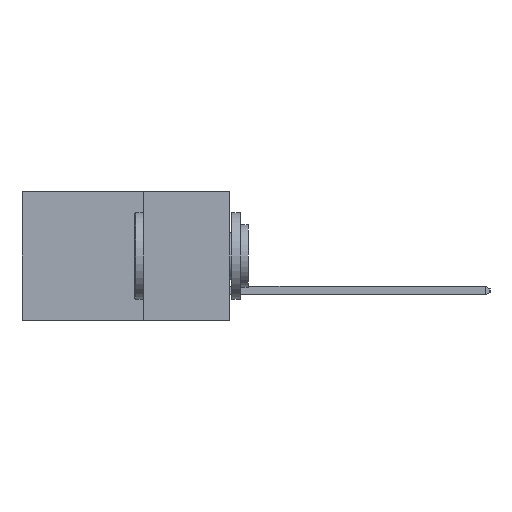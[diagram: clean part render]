
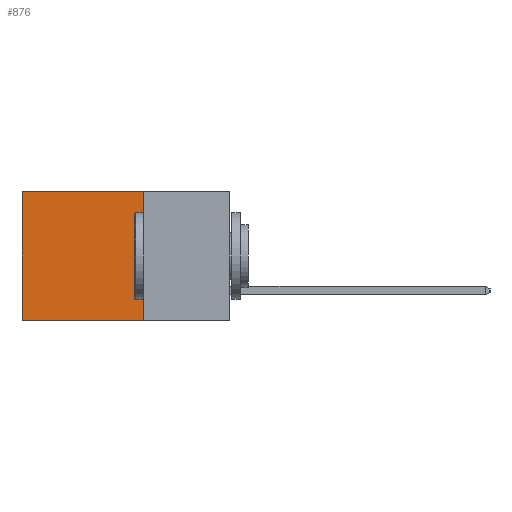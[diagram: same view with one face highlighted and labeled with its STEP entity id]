
A CAD part, left-side view. The second image highlights one B-rep face of the part: STEP entity #876.
In plain terms, the highlighted planar face has unit normal (-1, 0, 0).
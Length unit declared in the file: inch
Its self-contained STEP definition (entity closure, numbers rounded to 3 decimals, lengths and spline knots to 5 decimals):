
#803 = CARTESIAN_POINT ( 'NONE',  ( 0.298, 0.25, 0. ) ) ;
#833 = LINE ( 'NONE', #9248, #12348 ) ;
#876 = ADVANCED_FACE ( 'NONE', ( #4992 ), #11235, .F. ) ;
#1452 = EDGE_CURVE ( 'NONE', #3999, #16987, #19710, .T. ) ;
#1495 = EDGE_LOOP ( 'NONE', ( #12972, #16154, #17252, #1622 ) ) ;
#1622 = ORIENTED_EDGE ( 'NONE', *, *, #1452, .T. ) ;
#2278 = CARTESIAN_POINT ( 'NONE',  ( 0.298, 0.25, 0. ) ) ;
#2587 = VERTEX_POINT ( 'NONE', #16892 ) ;
#3330 = CARTESIAN_POINT ( 'NONE',  ( 0.298, 0.25, -0.37 ) ) ;
#3335 = CARTESIAN_POINT ( 'NONE',  ( 0.298, 0.25, -0.37 ) ) ;
#3428 = VECTOR ( 'NONE', #10988, 39.37008 ) ;
#3999 = VERTEX_POINT ( 'NONE', #2278 ) ;
#4008 = LINE ( 'NONE', #3335, #11269 ) ;
#4130 = DIRECTION ( 'NONE',  ( 0., 0., -1. ) ) ;
#4992 = FACE_OUTER_BOUND ( 'NONE', #1495, .T. ) ;
#5672 = CARTESIAN_POINT ( 'NONE',  ( 0.298, 0.6, 0. ) ) ;
#7982 = DIRECTION ( 'NONE',  ( 1., 0., 0. ) ) ;
#8150 = DIRECTION ( 'NONE',  ( 0., 0., -1. ) ) ;
#8777 = CARTESIAN_POINT ( 'NONE',  ( 0.298, 0.6, 0. ) ) ;
#9248 = CARTESIAN_POINT ( 'NONE',  ( 0.298, 0.25, 0. ) ) ;
#10777 = DIRECTION ( 'NONE',  ( 0., 0., -1. ) ) ;
#10870 = LINE ( 'NONE', #5672, #18910 ) ;
#10988 = DIRECTION ( 'NONE',  ( 0., 1., 0. ) ) ;
#11235 = PLANE ( 'NONE',  #14724 ) ;
#11269 = VECTOR ( 'NONE', #12668, 39.37008 ) ;
#11932 = EDGE_CURVE ( 'NONE', #15998, #2587, #4008, .T. ) ;
#12348 = VECTOR ( 'NONE', #10777, 39.37008 ) ;
#12668 = DIRECTION ( 'NONE',  ( 0., 1., 0. ) ) ;
#12972 = ORIENTED_EDGE ( 'NONE', *, *, #17650, .T. ) ;
#13404 = CARTESIAN_POINT ( 'NONE',  ( 0.298, 0.25, 0. ) ) ;
#14142 = EDGE_CURVE ( 'NONE', #3999, #15998, #833, .T. ) ;
#14724 = AXIS2_PLACEMENT_3D ( 'NONE', #13404, #7982, #8150 ) ;
#15998 = VERTEX_POINT ( 'NONE', #3330 ) ;
#16154 = ORIENTED_EDGE ( 'NONE', *, *, #11932, .F. ) ;
#16892 = CARTESIAN_POINT ( 'NONE',  ( 0.298, 0.6, -0.37 ) ) ;
#16987 = VERTEX_POINT ( 'NONE', #8777 ) ;
#17252 = ORIENTED_EDGE ( 'NONE', *, *, #14142, .F. ) ;
#17650 = EDGE_CURVE ( 'NONE', #16987, #2587, #10870, .T. ) ;
#18910 = VECTOR ( 'NONE', #4130, 39.37008 ) ;
#19710 = LINE ( 'NONE', #803, #3428 ) ;
